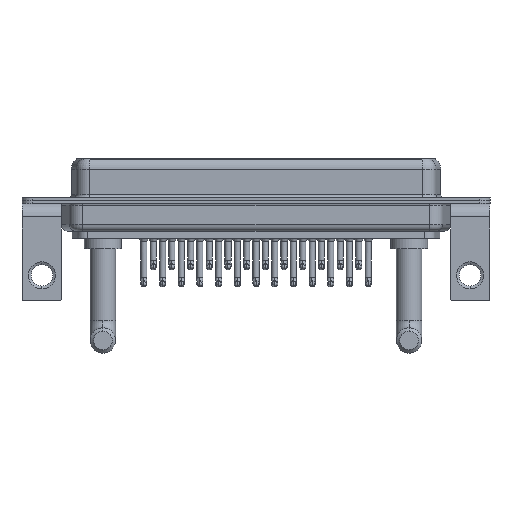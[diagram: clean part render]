
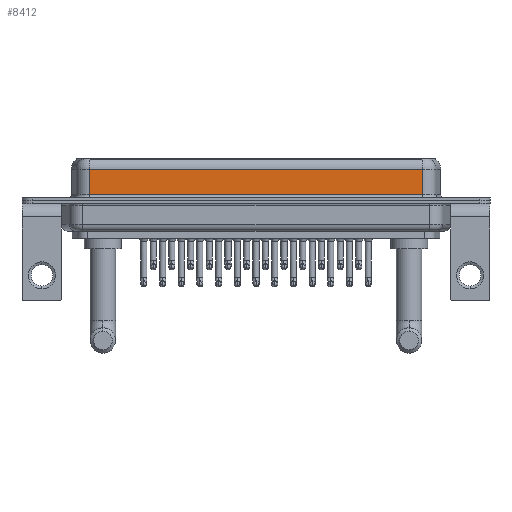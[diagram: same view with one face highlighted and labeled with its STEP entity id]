
A CAD part, front view. The second image highlights one B-rep face of the part: STEP entity #8412.
In plain terms, the highlighted planar face has unit normal (0, -1, 0).
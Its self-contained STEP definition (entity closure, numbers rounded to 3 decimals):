
#4390 = PLANE ( 'NONE',  #12067 ) ;
#5712 = EDGE_LOOP ( 'NONE', ( #12902, #20188, #25466, #6101 ) ) ;
#6101 = ORIENTED_EDGE ( 'NONE', *, *, #16995, .T. ) ;
#6146 = LINE ( 'NONE', #12349, #10407 ) ;
#6330 = DIRECTION ( 'NONE',  ( 0., 1., 0. ) ) ;
#7039 = LINE ( 'NONE', #24286, #17273 ) ;
#7333 = VECTOR ( 'NONE', #21084, 1000. ) ;
#8150 = CARTESIAN_POINT ( 'NONE',  ( 56.462, -3.95, 6.4 ) ) ;
#8412 = ADVANCED_FACE ( 'NONE', ( #14103 ), #4390, .F. ) ;
#8763 = VERTEX_POINT ( 'NONE', #16355 ) ;
#9293 = VERTEX_POINT ( 'NONE', #16201 ) ;
#9647 = LINE ( 'NONE', #17545, #12866 ) ;
#10407 = VECTOR ( 'NONE', #18050, 1000. ) ;
#11534 = CARTESIAN_POINT ( 'NONE',  ( 7.038, -3.95, 0.9 ) ) ;
#12039 = DIRECTION ( 'NONE',  ( 0., 0., 1. ) ) ;
#12067 = AXIS2_PLACEMENT_3D ( 'NONE', #8150, #6330, #12039 ) ;
#12349 = CARTESIAN_POINT ( 'NONE',  ( 56.462, -3.95, 6.4 ) ) ;
#12866 = VECTOR ( 'NONE', #24158, 1000. ) ;
#12902 = ORIENTED_EDGE ( 'NONE', *, *, #20884, .F. ) ;
#13146 = VERTEX_POINT ( 'NONE', #23667 ) ;
#14103 = FACE_OUTER_BOUND ( 'NONE', #5712, .T. ) ;
#16201 = CARTESIAN_POINT ( 'NONE',  ( 56.462, -3.95, 0.9 ) ) ;
#16355 = CARTESIAN_POINT ( 'NONE',  ( 7.038, -3.95, 4.65 ) ) ;
#16490 = DIRECTION ( 'NONE',  ( -1., 0., 0. ) ) ;
#16995 = EDGE_CURVE ( 'NONE', #18491, #9293, #25248, .T. ) ;
#17273 = VECTOR ( 'NONE', #16490, 1000. ) ;
#17545 = CARTESIAN_POINT ( 'NONE',  ( 7.038, -3.95, 6.4 ) ) ;
#17748 = EDGE_CURVE ( 'NONE', #13146, #8763, #7039, .T. ) ;
#18050 = DIRECTION ( 'NONE',  ( 0., 0., -1. ) ) ;
#18491 = VERTEX_POINT ( 'NONE', #11534 ) ;
#20188 = ORIENTED_EDGE ( 'NONE', *, *, #17748, .T. ) ;
#20884 = EDGE_CURVE ( 'NONE', #13146, #9293, #6146, .T. ) ;
#21084 = DIRECTION ( 'NONE',  ( 1., 0., 0. ) ) ;
#22120 = EDGE_CURVE ( 'NONE', #8763, #18491, #9647, .T. ) ;
#23041 = CARTESIAN_POINT ( 'NONE',  ( 56.462, -3.95, 0.9 ) ) ;
#23667 = CARTESIAN_POINT ( 'NONE',  ( 56.462, -3.95, 4.65 ) ) ;
#24158 = DIRECTION ( 'NONE',  ( 0., 0., -1. ) ) ;
#24286 = CARTESIAN_POINT ( 'NONE',  ( 56.462, -3.95, 4.65 ) ) ;
#25248 = LINE ( 'NONE', #23041, #7333 ) ;
#25466 = ORIENTED_EDGE ( 'NONE', *, *, #22120, .T. ) ;
